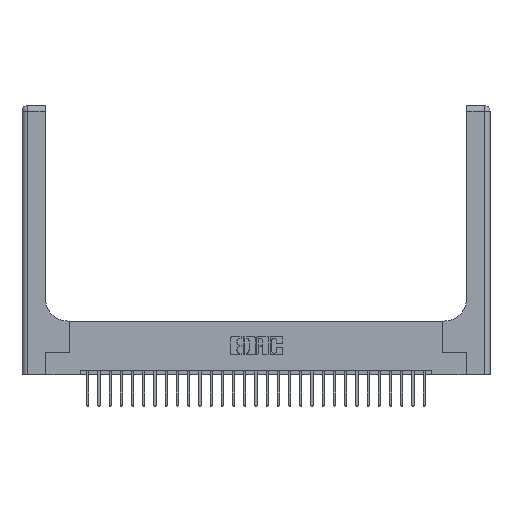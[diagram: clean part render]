
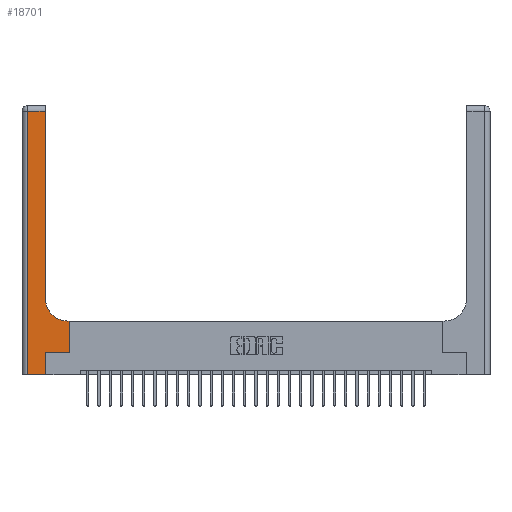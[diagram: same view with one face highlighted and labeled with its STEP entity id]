
A CAD part, top view. The second image highlights one B-rep face of the part: STEP entity #18701.
In plain terms, the highlighted planar face has unit normal (0, 0, 1).
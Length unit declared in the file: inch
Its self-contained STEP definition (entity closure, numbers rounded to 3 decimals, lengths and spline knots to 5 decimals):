
#543 = ORIENTED_EDGE ( 'NONE', *, *, #1412, .T. ) ;
#749 = CARTESIAN_POINT ( 'NONE',  ( 0.51, 0.6, 0.37 ) ) ;
#779 = EDGE_CURVE ( 'NONE', #3039, #14647, #4139, .T. ) ;
#803 = VERTEX_POINT ( 'NONE', #7163 ) ;
#1006 = CARTESIAN_POINT ( 'NONE',  ( 0.06, 2.94, 0.37 ) ) ;
#1319 = CARTESIAN_POINT ( 'NONE',  ( 0.265, 0.25, 0.37 ) ) ;
#1412 = EDGE_CURVE ( 'NONE', #21780, #16160, #19545, .T. ) ;
#1616 = LINE ( 'NONE', #6044, #18578 ) ;
#1831 = AXIS2_PLACEMENT_3D ( 'NONE', #15413, #4513, #9073 ) ;
#2088 = ORIENTED_EDGE ( 'NONE', *, *, #16970, .T. ) ;
#2283 = ORIENTED_EDGE ( 'NONE', *, *, #779, .T. ) ;
#2607 = CARTESIAN_POINT ( 'NONE',  ( 0.265, 0., 0.37 ) ) ;
#3039 = VERTEX_POINT ( 'NONE', #5404 ) ;
#3297 = VECTOR ( 'NONE', #3538, 39.37008 ) ;
#3538 = DIRECTION ( 'NONE',  ( -1., 0., 0. ) ) ;
#3958 = EDGE_CURVE ( 'NONE', #803, #24088, #10032, .T. ) ;
#4139 = LINE ( 'NONE', #2607, #5836 ) ;
#4310 = VECTOR ( 'NONE', #5484, 39.37008 ) ;
#4513 = DIRECTION ( 'NONE',  ( 0., 0., -1. ) ) ;
#4910 = CARTESIAN_POINT ( 'NONE',  ( 0.26, 3., 0.37 ) ) ;
#5404 = CARTESIAN_POINT ( 'NONE',  ( 0.265, 0., 0.37 ) ) ;
#5484 = DIRECTION ( 'NONE',  ( 1., 0., 0. ) ) ;
#5497 = VERTEX_POINT ( 'NONE', #22996 ) ;
#5836 = VECTOR ( 'NONE', #16820, 39.37008 ) ;
#6044 = CARTESIAN_POINT ( 'NONE',  ( 0., 2.94, 0.37 ) ) ;
#6608 = DIRECTION ( 'NONE',  ( 0., 0., -1. ) ) ;
#6949 = VECTOR ( 'NONE', #13350, 39.37008 ) ;
#7149 = CIRCLE ( 'NONE', #1831, 0.25 ) ;
#7163 = CARTESIAN_POINT ( 'NONE',  ( 0.528, 0.6, 0.37 ) ) ;
#7422 = DIRECTION ( 'NONE',  ( 0., 1., 0. ) ) ;
#7930 = CARTESIAN_POINT ( 'NONE',  ( 0.26, 2.94, 0.37 ) ) ;
#8959 = CARTESIAN_POINT ( 'NONE',  ( 0., 3., 0.37 ) ) ;
#9073 = DIRECTION ( 'NONE',  ( 1., 0., 0. ) ) ;
#9348 = LINE ( 'NONE', #20625, #14604 ) ;
#10032 = LINE ( 'NONE', #14446, #3297 ) ;
#11485 = CARTESIAN_POINT ( 'NONE',  ( 0.265, 0.25, 0.37 ) ) ;
#11958 = VECTOR ( 'NONE', #22772, 39.37008 ) ;
#12329 = EDGE_CURVE ( 'NONE', #5497, #3039, #9348, .T. ) ;
#12643 = ORIENTED_EDGE ( 'NONE', *, *, #3958, .T. ) ;
#13350 = DIRECTION ( 'NONE',  ( 0., 1., 0. ) ) ;
#13405 = EDGE_CURVE ( 'NONE', #16160, #26745, #1616, .T. ) ;
#13524 = CARTESIAN_POINT ( 'NONE',  ( 0.26, 0.85, 0.37 ) ) ;
#13647 = LINE ( 'NONE', #1319, #4310 ) ;
#14340 = LINE ( 'NONE', #19997, #11958 ) ;
#14446 = CARTESIAN_POINT ( 'NONE',  ( 0.26, 0.6, 0.37 ) ) ;
#14604 = VECTOR ( 'NONE', #24134, 39.37008 ) ;
#14647 = VERTEX_POINT ( 'NONE', #11485 ) ;
#14679 = ORIENTED_EDGE ( 'NONE', *, *, #12329, .T. ) ;
#15413 = CARTESIAN_POINT ( 'NONE',  ( 0.51, 0.85, 0.37 ) ) ;
#15784 = AXIS2_PLACEMENT_3D ( 'NONE', #8959, #6608, #23747 ) ;
#16160 = VERTEX_POINT ( 'NONE', #7930 ) ;
#16520 = VECTOR ( 'NONE', #7422, 39.37008 ) ;
#16820 = DIRECTION ( 'NONE',  ( 0., 1., 0. ) ) ;
#16970 = EDGE_CURVE ( 'NONE', #18753, #803, #21934, .T. ) ;
#17228 = FACE_OUTER_BOUND ( 'NONE', #25524, .T. ) ;
#18578 = VECTOR ( 'NONE', #18875, 39.37008 ) ;
#18701 = ADVANCED_FACE ( 'NONE', ( #17228 ), #21943, .F. ) ;
#18753 = VERTEX_POINT ( 'NONE', #21403 ) ;
#18868 = EDGE_CURVE ( 'NONE', #14647, #18753, #13647, .T. ) ;
#18875 = DIRECTION ( 'NONE',  ( -1., 0., 0. ) ) ;
#19545 = LINE ( 'NONE', #4910, #6949 ) ;
#19997 = CARTESIAN_POINT ( 'NONE',  ( 0.06, 3., 0.37 ) ) ;
#20625 = CARTESIAN_POINT ( 'NONE',  ( 0., 0., 0.37 ) ) ;
#21403 = CARTESIAN_POINT ( 'NONE',  ( 0.528, 0.25, 0.37 ) ) ;
#21726 = ORIENTED_EDGE ( 'NONE', *, *, #23989, .T. ) ;
#21780 = VERTEX_POINT ( 'NONE', #13524 ) ;
#21934 = LINE ( 'NONE', #22202, #16520 ) ;
#21943 = PLANE ( 'NONE',  #15784 ) ;
#22202 = CARTESIAN_POINT ( 'NONE',  ( 0.528, 0.25, 0.37 ) ) ;
#22772 = DIRECTION ( 'NONE',  ( 0., -1., 0. ) ) ;
#22870 = ORIENTED_EDGE ( 'NONE', *, *, #25059, .T. ) ;
#22996 = CARTESIAN_POINT ( 'NONE',  ( 0.06, 0., 0.37 ) ) ;
#23688 = ORIENTED_EDGE ( 'NONE', *, *, #13405, .T. ) ;
#23747 = DIRECTION ( 'NONE',  ( -1., 0., 0. ) ) ;
#23989 = EDGE_CURVE ( 'NONE', #24088, #21780, #7149, .T. ) ;
#24088 = VERTEX_POINT ( 'NONE', #749 ) ;
#24134 = DIRECTION ( 'NONE',  ( 1., 0., 0. ) ) ;
#24848 = ORIENTED_EDGE ( 'NONE', *, *, #18868, .T. ) ;
#25059 = EDGE_CURVE ( 'NONE', #26745, #5497, #14340, .T. ) ;
#25524 = EDGE_LOOP ( 'NONE', ( #543, #23688, #22870, #14679, #2283, #24848, #2088, #12643, #21726 ) ) ;
#26745 = VERTEX_POINT ( 'NONE', #1006 ) ;
